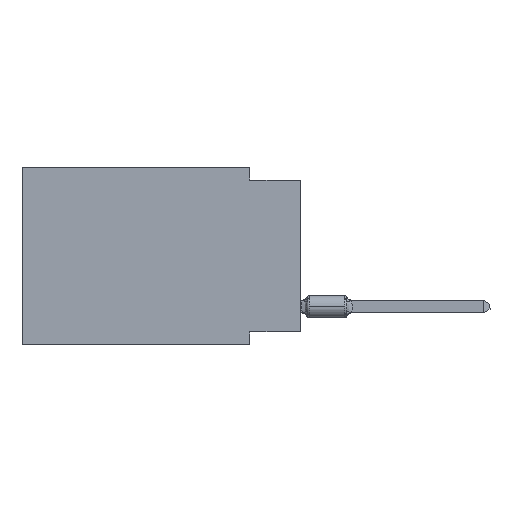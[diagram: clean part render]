
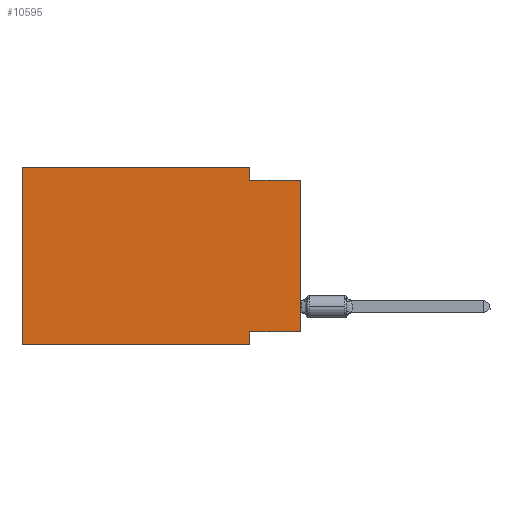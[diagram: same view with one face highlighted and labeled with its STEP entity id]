
A CAD part, left-side view. The second image highlights one B-rep face of the part: STEP entity #10595.
In plain terms, the highlighted planar face has unit normal (-1, 0, 0).
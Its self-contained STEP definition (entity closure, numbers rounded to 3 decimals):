
#133 = EDGE_CURVE ( 'NONE', #17389, #16898, #13851, .T. ) ;
#619 = DIRECTION ( 'NONE',  ( 0., -1., 0. ) ) ;
#765 = VECTOR ( 'NONE', #12756, 1000. ) ;
#814 = CARTESIAN_POINT ( 'NONE',  ( 0., 13.97, 0. ) ) ;
#1081 = CARTESIAN_POINT ( 'NONE',  ( 0., 0., -0.635 ) ) ;
#1448 = ORIENTED_EDGE ( 'NONE', *, *, #9854, .F. ) ;
#1985 = DIRECTION ( 'NONE',  ( 0., 0., -1. ) ) ;
#2270 = EDGE_CURVE ( 'NONE', #13502, #10487, #9543, .T. ) ;
#3055 = CARTESIAN_POINT ( 'NONE',  ( 0., 13.97, 0. ) ) ;
#3595 = VECTOR ( 'NONE', #19584, 1000. ) ;
#3610 = CARTESIAN_POINT ( 'NONE',  ( 0., 13.97, -8.89 ) ) ;
#3679 = VECTOR ( 'NONE', #16769, 1000. ) ;
#3695 = VERTEX_POINT ( 'NONE', #12545 ) ;
#3809 = FACE_OUTER_BOUND ( 'NONE', #12028, .T. ) ;
#4068 = VECTOR ( 'NONE', #17410, 1000. ) ;
#4258 = ORIENTED_EDGE ( 'NONE', *, *, #5871, .F. ) ;
#4530 = LINE ( 'NONE', #9071, #3595 ) ;
#4722 = DIRECTION ( 'NONE',  ( 0., -1., 0. ) ) ;
#5011 = CARTESIAN_POINT ( 'NONE',  ( 0., 13.97, -8.89 ) ) ;
#5354 = ORIENTED_EDGE ( 'NONE', *, *, #9945, .F. ) ;
#5387 = DIRECTION ( 'NONE',  ( 0., 0., -1. ) ) ;
#5871 = EDGE_CURVE ( 'NONE', #3695, #9277, #11339, .T. ) ;
#6133 = LINE ( 'NONE', #3055, #3679 ) ;
#6212 = CARTESIAN_POINT ( 'NONE',  ( 0., 0., -0.635 ) ) ;
#6782 = CARTESIAN_POINT ( 'NONE',  ( 0., 13.97, 0. ) ) ;
#7282 = VECTOR ( 'NONE', #619, 1000. ) ;
#7441 = EDGE_CURVE ( 'NONE', #9277, #12864, #9554, .T. ) ;
#7450 = EDGE_CURVE ( 'NONE', #13772, #10487, #14227, .T. ) ;
#7620 = AXIS2_PLACEMENT_3D ( 'NONE', #6782, #9841, #5387 ) ;
#9071 = CARTESIAN_POINT ( 'NONE',  ( 0., 0., -8.255 ) ) ;
#9277 = VERTEX_POINT ( 'NONE', #16066 ) ;
#9543 = LINE ( 'NONE', #15602, #16344 ) ;
#9554 = LINE ( 'NONE', #15718, #12025 ) ;
#9652 = DIRECTION ( 'NONE',  ( 0., 0., -1. ) ) ;
#9841 = DIRECTION ( 'NONE',  ( 1., 0., 0. ) ) ;
#9854 = EDGE_CURVE ( 'NONE', #17389, #13502, #4530, .T. ) ;
#9945 = EDGE_CURVE ( 'NONE', #12864, #16898, #16554, .T. ) ;
#10487 = VERTEX_POINT ( 'NONE', #15819 ) ;
#10595 = ADVANCED_FACE ( 'NONE', ( #3809 ), #16214, .F. ) ;
#11339 = LINE ( 'NONE', #814, #4068 ) ;
#12025 = VECTOR ( 'NONE', #9652, 1000. ) ;
#12028 = EDGE_LOOP ( 'NONE', ( #12292, #5354, #17263, #4258, #15725, #17534, #14821, #1448 ) ) ;
#12292 = ORIENTED_EDGE ( 'NONE', *, *, #133, .T. ) ;
#12545 = CARTESIAN_POINT ( 'NONE',  ( 0., 13.97, 0. ) ) ;
#12552 = CARTESIAN_POINT ( 'NONE',  ( 0., 0., 0. ) ) ;
#12756 = DIRECTION ( 'NONE',  ( 0., 0., 1. ) ) ;
#12864 = VERTEX_POINT ( 'NONE', #15828 ) ;
#13091 = VECTOR ( 'NONE', #4722, 1000. ) ;
#13502 = VERTEX_POINT ( 'NONE', #17439 ) ;
#13772 = VERTEX_POINT ( 'NONE', #5011 ) ;
#13851 = LINE ( 'NONE', #12552, #765 ) ;
#14227 = LINE ( 'NONE', #3610, #7282 ) ;
#14821 = ORIENTED_EDGE ( 'NONE', *, *, #2270, .F. ) ;
#15602 = CARTESIAN_POINT ( 'NONE',  ( 0., 2.54, -8.89 ) ) ;
#15718 = CARTESIAN_POINT ( 'NONE',  ( 0., 2.54, 0. ) ) ;
#15725 = ORIENTED_EDGE ( 'NONE', *, *, #17401, .F. ) ;
#15819 = CARTESIAN_POINT ( 'NONE',  ( 0., 2.54, -8.89 ) ) ;
#15828 = CARTESIAN_POINT ( 'NONE',  ( 0., 2.54, -0.635 ) ) ;
#16066 = CARTESIAN_POINT ( 'NONE',  ( 0., 2.54, 0. ) ) ;
#16214 = PLANE ( 'NONE',  #7620 ) ;
#16344 = VECTOR ( 'NONE', #1985, 1000. ) ;
#16554 = LINE ( 'NONE', #6212, #13091 ) ;
#16676 = CARTESIAN_POINT ( 'NONE',  ( 0., 0., -8.255 ) ) ;
#16769 = DIRECTION ( 'NONE',  ( 0., 0., 1. ) ) ;
#16898 = VERTEX_POINT ( 'NONE', #1081 ) ;
#17263 = ORIENTED_EDGE ( 'NONE', *, *, #7441, .F. ) ;
#17389 = VERTEX_POINT ( 'NONE', #16676 ) ;
#17401 = EDGE_CURVE ( 'NONE', #13772, #3695, #6133, .T. ) ;
#17410 = DIRECTION ( 'NONE',  ( 0., -1., 0. ) ) ;
#17439 = CARTESIAN_POINT ( 'NONE',  ( 0., 2.54, -8.255 ) ) ;
#17534 = ORIENTED_EDGE ( 'NONE', *, *, #7450, .T. ) ;
#19584 = DIRECTION ( 'NONE',  ( 0., 1., 0. ) ) ;
